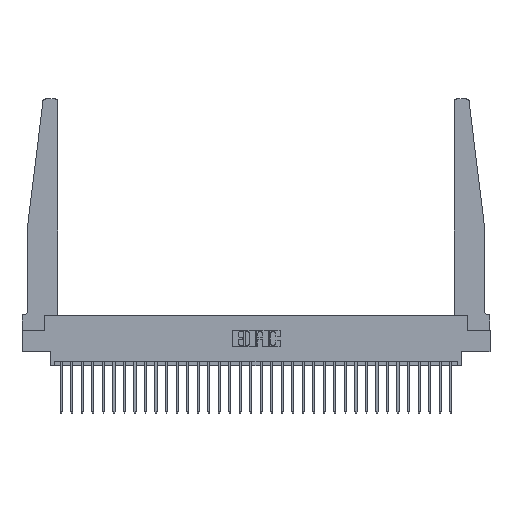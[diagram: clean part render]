
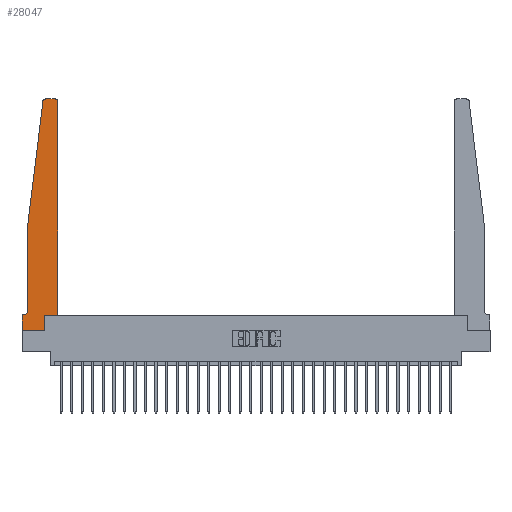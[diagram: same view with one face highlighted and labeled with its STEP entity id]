
A CAD part, top view. The second image highlights one B-rep face of the part: STEP entity #28047.
In plain terms, the highlighted planar face has unit normal (0, 0, 1).
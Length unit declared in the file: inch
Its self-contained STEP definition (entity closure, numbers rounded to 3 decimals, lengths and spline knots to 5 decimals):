
#4 = CARTESIAN_POINT ( 'NONE',  ( 0.2605, 0.18, 0.37 ) ) ;
#64 = CARTESIAN_POINT ( 'NONE',  ( 0.065, 1.25, 0.37 ) ) ;
#149 = EDGE_CURVE ( 'NONE', #13328, #24282, #19817, .T. ) ;
#173 = LINE ( 'NONE', #25071, #18149 ) ;
#198 = EDGE_CURVE ( 'NONE', #22602, #14079, #6574, .T. ) ;
#297 = AXIS2_PLACEMENT_3D ( 'NONE', #17921, #3856, #20277 ) ;
#447 = DIRECTION ( 'NONE',  ( 0., -1., 0. ) ) ;
#453 = ORIENTED_EDGE ( 'NONE', *, *, #2646, .T. ) ;
#564 = LINE ( 'NONE', #24142, #19291 ) ;
#714 = VERTEX_POINT ( 'NONE', #6569 ) ;
#2646 = EDGE_CURVE ( 'NONE', #14079, #714, #11584, .T. ) ;
#2734 = CARTESIAN_POINT ( 'NONE',  ( 0.2605, 0., 0.37 ) ) ;
#3519 = EDGE_CURVE ( 'NONE', #15726, #22602, #564, .T. ) ;
#3856 = DIRECTION ( 'NONE',  ( 0., 0., 1. ) ) ;
#3988 = CIRCLE ( 'NONE', #297, 0.03 ) ;
#4840 = ORIENTED_EDGE ( 'NONE', *, *, #3519, .T. ) ;
#5045 = ORIENTED_EDGE ( 'NONE', *, *, #9958, .T. ) ;
#5574 = VERTEX_POINT ( 'NONE', #11334 ) ;
#5793 = VERTEX_POINT ( 'NONE', #2734 ) ;
#6006 = ORIENTED_EDGE ( 'NONE', *, *, #19001, .T. ) ;
#6182 = PLANE ( 'NONE',  #12419 ) ;
#6186 = CARTESIAN_POINT ( 'NONE',  ( 0.395, 2.75, 0.37 ) ) ;
#6201 = VERTEX_POINT ( 'NONE', #20670 ) ;
#6569 = CARTESIAN_POINT ( 'NONE',  ( 0.27653, 2.75, 0.37 ) ) ;
#6574 = CIRCLE ( 'NONE', #19021, 0.03 ) ;
#7242 = ORIENTED_EDGE ( 'NONE', *, *, #18036, .T. ) ;
#7309 = DIRECTION ( 'NONE',  ( 0., 0., 1. ) ) ;
#7549 = CARTESIAN_POINT ( 'NONE',  ( 0.015, 0.2375, 0.37 ) ) ;
#7737 = EDGE_CURVE ( 'NONE', #714, #13328, #3988, .T. ) ;
#7908 = LINE ( 'NONE', #12232, #20424 ) ;
#8537 = DIRECTION ( 'NONE',  ( 1., 0., 0. ) ) ;
#8771 = ORIENTED_EDGE ( 'NONE', *, *, #9410, .T. ) ;
#9410 = EDGE_CURVE ( 'NONE', #24282, #5574, #9431, .T. ) ;
#9431 = LINE ( 'NONE', #28832, #27373 ) ;
#9907 = DIRECTION ( 'NONE',  ( -1., 0., 0. ) ) ;
#9958 = EDGE_CURVE ( 'NONE', #22032, #5793, #7908, .T. ) ;
#9962 = AXIS2_PLACEMENT_3D ( 'NONE', #7549, #23994, #9907 ) ;
#10068 = DIRECTION ( 'NONE',  ( 0., 1., 0. ) ) ;
#10505 = CARTESIAN_POINT ( 'NONE',  ( 0.425, 2.72, 0.37 ) ) ;
#11292 = EDGE_CURVE ( 'NONE', #5793, #28333, #24026, .T. ) ;
#11334 = CARTESIAN_POINT ( 'NONE',  ( 0.065, 0.2375, 0.37 ) ) ;
#11584 = LINE ( 'NONE', #13816, #29523 ) ;
#11925 = VECTOR ( 'NONE', #19597, 39.37008 ) ;
#11956 = CARTESIAN_POINT ( 'NONE',  ( 0.065, 1.25, 0.37 ) ) ;
#12232 = CARTESIAN_POINT ( 'NONE',  ( 0., 0., 0.37 ) ) ;
#12419 = AXIS2_PLACEMENT_3D ( 'NONE', #13137, #22621, #8537 ) ;
#12478 = CARTESIAN_POINT ( 'NONE',  ( 0.425, 0.18, 0.37 ) ) ;
#13137 = CARTESIAN_POINT ( 'NONE',  ( 0., 0.1875, 0.37 ) ) ;
#13328 = VERTEX_POINT ( 'NONE', #26236 ) ;
#13373 = DIRECTION ( 'NONE',  ( -1., 0., 0. ) ) ;
#13684 = ORIENTED_EDGE ( 'NONE', *, *, #14488, .T. ) ;
#13816 = CARTESIAN_POINT ( 'NONE',  ( 0.25, 2.75, 0.37 ) ) ;
#13954 = VECTOR ( 'NONE', #447, 39.37008 ) ;
#14079 = VERTEX_POINT ( 'NONE', #6186 ) ;
#14488 = EDGE_CURVE ( 'NONE', #15586, #22032, #20193, .T. ) ;
#15395 = EDGE_LOOP ( 'NONE', ( #453, #19104, #16856, #8771, #26163, #6006, #13684, #5045, #29624, #7242, #4840, #25875 ) ) ;
#15586 = VERTEX_POINT ( 'NONE', #16396 ) ;
#15726 = VERTEX_POINT ( 'NONE', #17007 ) ;
#16396 = CARTESIAN_POINT ( 'NONE',  ( 0., 0.1875, 0.37 ) ) ;
#16477 = DIRECTION ( 'NONE',  ( -0.122, -0.992, 0. ) ) ;
#16856 = ORIENTED_EDGE ( 'NONE', *, *, #149, .T. ) ;
#17007 = CARTESIAN_POINT ( 'NONE',  ( 0.425, 0.18, 0.37 ) ) ;
#17921 = CARTESIAN_POINT ( 'NONE',  ( 0.27653, 2.72, 0.37 ) ) ;
#18036 = EDGE_CURVE ( 'NONE', #28333, #15726, #18203, .T. ) ;
#18149 = VECTOR ( 'NONE', #13373, 39.37008 ) ;
#18203 = LINE ( 'NONE', #12478, #11925 ) ;
#19001 = EDGE_CURVE ( 'NONE', #6201, #15586, #173, .T. ) ;
#19021 = AXIS2_PLACEMENT_3D ( 'NONE', #21410, #7309, #23761 ) ;
#19104 = ORIENTED_EDGE ( 'NONE', *, *, #7737, .T. ) ;
#19291 = VECTOR ( 'NONE', #10068, 39.37008 ) ;
#19597 = DIRECTION ( 'NONE',  ( 1., 0., 0. ) ) ;
#19817 = LINE ( 'NONE', #64, #25303 ) ;
#20193 = LINE ( 'NONE', #26165, #13954 ) ;
#20277 = DIRECTION ( 'NONE',  ( 1., 0., 0. ) ) ;
#20424 = VECTOR ( 'NONE', #28599, 39.37008 ) ;
#20670 = CARTESIAN_POINT ( 'NONE',  ( 0.015, 0.1875, 0.37 ) ) ;
#21056 = CARTESIAN_POINT ( 'NONE',  ( 0.2605, 0.18, 0.37 ) ) ;
#21410 = CARTESIAN_POINT ( 'NONE',  ( 0.395, 2.72, 0.37 ) ) ;
#21589 = EDGE_CURVE ( 'NONE', #5574, #6201, #27894, .T. ) ;
#22032 = VERTEX_POINT ( 'NONE', #27233 ) ;
#22550 = VECTOR ( 'NONE', #23489, 39.37008 ) ;
#22602 = VERTEX_POINT ( 'NONE', #10505 ) ;
#22621 = DIRECTION ( 'NONE',  ( 0., 0., 1. ) ) ;
#23489 = DIRECTION ( 'NONE',  ( 0., 1., 0. ) ) ;
#23761 = DIRECTION ( 'NONE',  ( 1., 0., 0. ) ) ;
#23994 = DIRECTION ( 'NONE',  ( 0., 0., -1. ) ) ;
#24026 = LINE ( 'NONE', #4, #22550 ) ;
#24142 = CARTESIAN_POINT ( 'NONE',  ( 0.425, 0.18, 0.37 ) ) ;
#24282 = VERTEX_POINT ( 'NONE', #11956 ) ;
#24289 = DIRECTION ( 'NONE',  ( 0., -1., 0. ) ) ;
#25071 = CARTESIAN_POINT ( 'NONE',  ( 0.065, 0.1875, 0.37 ) ) ;
#25303 = VECTOR ( 'NONE', #16477, 39.37008 ) ;
#25492 = DIRECTION ( 'NONE',  ( -1., 0., 0. ) ) ;
#25875 = ORIENTED_EDGE ( 'NONE', *, *, #198, .T. ) ;
#26163 = ORIENTED_EDGE ( 'NONE', *, *, #21589, .T. ) ;
#26165 = CARTESIAN_POINT ( 'NONE',  ( 0., 0., 0.37 ) ) ;
#26236 = CARTESIAN_POINT ( 'NONE',  ( 0.24675, 2.72367, 0.37 ) ) ;
#27233 = CARTESIAN_POINT ( 'NONE',  ( 0., 0., 0.37 ) ) ;
#27373 = VECTOR ( 'NONE', #24289, 39.37008 ) ;
#27510 = FACE_OUTER_BOUND ( 'NONE', #15395, .T. ) ;
#27894 = CIRCLE ( 'NONE', #9962, 0.05 ) ;
#28047 = ADVANCED_FACE ( 'NONE', ( #27510 ), #6182, .T. ) ;
#28333 = VERTEX_POINT ( 'NONE', #21056 ) ;
#28599 = DIRECTION ( 'NONE',  ( 1., 0., 0. ) ) ;
#28832 = CARTESIAN_POINT ( 'NONE',  ( 0.065, 1.25, 0.37 ) ) ;
#29523 = VECTOR ( 'NONE', #25492, 39.37008 ) ;
#29624 = ORIENTED_EDGE ( 'NONE', *, *, #11292, .T. ) ;
